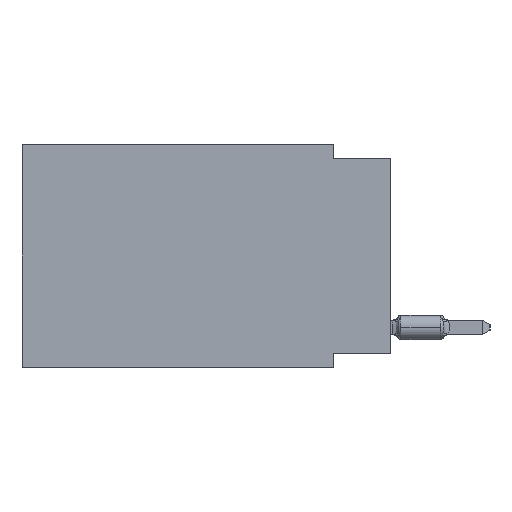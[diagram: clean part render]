
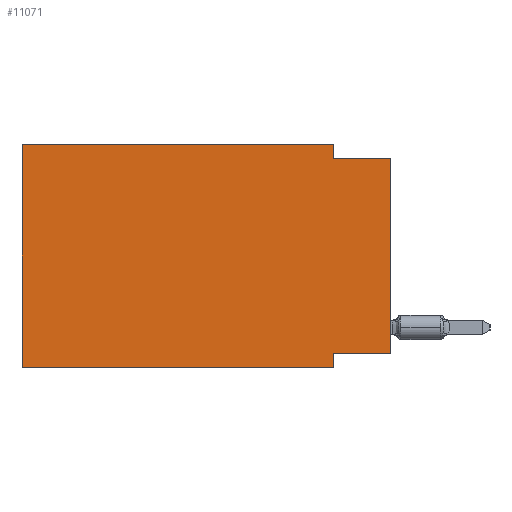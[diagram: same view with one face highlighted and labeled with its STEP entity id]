
A CAD part, left-side view. The second image highlights one B-rep face of the part: STEP entity #11071.
In plain terms, the highlighted planar face has unit normal (-1, 0, 0).
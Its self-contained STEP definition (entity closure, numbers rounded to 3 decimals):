
#1291 = ORIENTED_EDGE ( 'NONE', *, *, #65539, .F. ) ;
#6022 = DIRECTION ( 'NONE',  ( 0., -1., 0. ) ) ;
#7191 = ORIENTED_EDGE ( 'NONE', *, *, #65025, .T. ) ;
#7683 = ORIENTED_EDGE ( 'NONE', *, *, #15436, .F. ) ;
#8007 = CARTESIAN_POINT ( 'NONE',  ( 0., 16.383, 0. ) ) ;
#8328 = FACE_OUTER_BOUND ( 'NONE', #12533, .T. ) ;
#8384 = VERTEX_POINT ( 'NONE', #9307 ) ;
#9247 = VECTOR ( 'NONE', #66214, 1000. ) ;
#9307 = CARTESIAN_POINT ( 'NONE',  ( 0., 16.383, 0. ) ) ;
#10391 = DIRECTION ( 'NONE',  ( 0., 1., 0. ) ) ;
#10901 = ORIENTED_EDGE ( 'NONE', *, *, #18740, .F. ) ;
#11071 = ADVANCED_FACE ( 'NONE', ( #8328 ), #37489, .F. ) ;
#11280 = CARTESIAN_POINT ( 'NONE',  ( 0., 2.54, -0.635 ) ) ;
#12533 = EDGE_LOOP ( 'NONE', ( #31367, #40726, #1291, #10901, #7683, #7191, #55250, #39594 ) ) ;
#13088 = DIRECTION ( 'NONE',  ( 0., -1., 0. ) ) ;
#15074 = LINE ( 'NONE', #31135, #54253 ) ;
#15436 = EDGE_CURVE ( 'NONE', #65180, #8384, #65463, .T. ) ;
#17767 = DIRECTION ( 'NONE',  ( 0., -1., 0. ) ) ;
#18611 = VECTOR ( 'NONE', #6022, 1000. ) ;
#18740 = EDGE_CURVE ( 'NONE', #8384, #63033, #57981, .T. ) ;
#19150 = CARTESIAN_POINT ( 'NONE',  ( 0., 0., 0. ) ) ;
#20318 = VERTEX_POINT ( 'NONE', #46209 ) ;
#21963 = VERTEX_POINT ( 'NONE', #36723 ) ;
#24589 = EDGE_CURVE ( 'NONE', #21963, #44552, #65337, .T. ) ;
#30007 = VECTOR ( 'NONE', #17767, 1000. ) ;
#31135 = CARTESIAN_POINT ( 'NONE',  ( 0., 0., -9.271 ) ) ;
#31367 = ORIENTED_EDGE ( 'NONE', *, *, #24589, .T. ) ;
#32703 = DIRECTION ( 'NONE',  ( 0., 0., -1. ) ) ;
#32837 = CARTESIAN_POINT ( 'NONE',  ( 0., 2.54, 0. ) ) ;
#35087 = CARTESIAN_POINT ( 'NONE',  ( 0., 2.54, 0. ) ) ;
#36069 = CARTESIAN_POINT ( 'NONE',  ( 0., 0., -0.635 ) ) ;
#36723 = CARTESIAN_POINT ( 'NONE',  ( 0., 0., -9.271 ) ) ;
#37018 = VECTOR ( 'NONE', #13088, 1000. ) ;
#37254 = VECTOR ( 'NONE', #55974, 1000. ) ;
#37489 = PLANE ( 'NONE',  #37867 ) ;
#37867 = AXIS2_PLACEMENT_3D ( 'NONE', #8007, #62914, #63902 ) ;
#39594 = ORIENTED_EDGE ( 'NONE', *, *, #40417, .F. ) ;
#40417 = EDGE_CURVE ( 'NONE', #21963, #20318, #15074, .T. ) ;
#40644 = CARTESIAN_POINT ( 'NONE',  ( 0., 2.54, -9.906 ) ) ;
#40726 = ORIENTED_EDGE ( 'NONE', *, *, #62241, .F. ) ;
#44552 = VERTEX_POINT ( 'NONE', #36069 ) ;
#44726 = EDGE_CURVE ( 'NONE', #20318, #53470, #53471, .T. ) ;
#44745 = CARTESIAN_POINT ( 'NONE',  ( 0., 16.383, 0. ) ) ;
#46209 = CARTESIAN_POINT ( 'NONE',  ( 0., 2.54, -9.271 ) ) ;
#51908 = LINE ( 'NONE', #56928, #18611 ) ;
#53470 = VERTEX_POINT ( 'NONE', #40644 ) ;
#53471 = LINE ( 'NONE', #58170, #60150 ) ;
#54253 = VECTOR ( 'NONE', #10391, 1000. ) ;
#54623 = CARTESIAN_POINT ( 'NONE',  ( 0., 16.383, -9.906 ) ) ;
#55250 = ORIENTED_EDGE ( 'NONE', *, *, #44726, .F. ) ;
#55974 = DIRECTION ( 'NONE',  ( 0., 0., 1. ) ) ;
#56928 = CARTESIAN_POINT ( 'NONE',  ( 0., 0., -0.635 ) ) ;
#57981 = LINE ( 'NONE', #62330, #30007 ) ;
#58170 = CARTESIAN_POINT ( 'NONE',  ( 0., 2.54, -9.906 ) ) ;
#58971 = LINE ( 'NONE', #54623, #37018 ) ;
#59144 = DIRECTION ( 'NONE',  ( 0., 0., 1. ) ) ;
#60150 = VECTOR ( 'NONE', #32703, 1000. ) ;
#61006 = VERTEX_POINT ( 'NONE', #11280 ) ;
#62241 = EDGE_CURVE ( 'NONE', #61006, #44552, #51908, .T. ) ;
#62330 = CARTESIAN_POINT ( 'NONE',  ( 0., 16.383, 0. ) ) ;
#62914 = DIRECTION ( 'NONE',  ( 1., 0., 0. ) ) ;
#63033 = VERTEX_POINT ( 'NONE', #32837 ) ;
#63902 = DIRECTION ( 'NONE',  ( 0., 0., -1. ) ) ;
#64902 = LINE ( 'NONE', #35087, #9247 ) ;
#64971 = CARTESIAN_POINT ( 'NONE',  ( 0., 16.383, -9.906 ) ) ;
#65025 = EDGE_CURVE ( 'NONE', #65180, #53470, #58971, .T. ) ;
#65083 = VECTOR ( 'NONE', #59144, 1000. ) ;
#65180 = VERTEX_POINT ( 'NONE', #64971 ) ;
#65337 = LINE ( 'NONE', #19150, #37254 ) ;
#65463 = LINE ( 'NONE', #44745, #65083 ) ;
#65539 = EDGE_CURVE ( 'NONE', #63033, #61006, #64902, .T. ) ;
#66214 = DIRECTION ( 'NONE',  ( 0., 0., -1. ) ) ;
